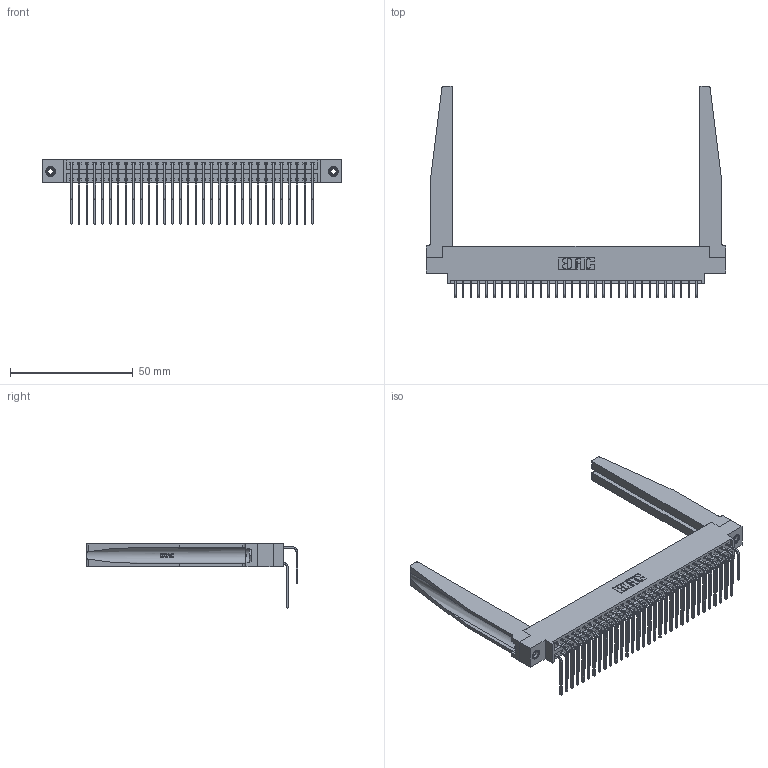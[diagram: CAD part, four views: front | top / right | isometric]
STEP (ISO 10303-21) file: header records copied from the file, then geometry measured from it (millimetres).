
FILE_DESCRIPTION (( 'STEP AP203' ), '1' );
FILE_NAME ('346-064-559-878.STEP', '2022-05-24T16:17:26', ( '' ), ( '' ), 'SwSTEP 2.0', 'SolidWorks 2020', '' );
FILE_SCHEMA (( 'CONFIG_CONTROL_DESIGN' ));
Length unit declared in the file: inch
Products named in the file (6): 346-220-078_345-220-078; 346-064-559-878; 346 Part_0.170 Offset - 0.156 Dia-TH; 345-250-001_345-250-001-102; 345-292-001_558 559 Tail - 1; 345-292-001_559 Tail - 2
Assembly tree (69 placements, depth 2):
  346-064-559-878
    346 Part_0.170 Offset - 0.156 Dia-TH
    345-292-001_558 559 Tail - 1  x32
    345-292-001_559 Tail - 2  x32
    346-220-078_345-220-078  x2
    345-250-001_345-250-001-102  x2
Bounding box: 122.17 x 86.17 x 26.16 mm (x, y, z)
Volume: 18941.2 mm3; surface area: 24904.9 mm2
Topology: 69 solids, 69 shells, 3830 faces, 11289 edges, 7430 vertices
Faces by surface type: plane 2604, cylinder 1174, bspline 36, cone 12, torus 4
Entity records: 29310 total; most frequent: CARTESIAN_POINT 5840, ORIENTED_EDGE 4610, DIRECTION 4155, EDGE_CURVE 2305, VECTOR 1911, LINE 1911, VERTEX_POINT 1528, AXIS2_PLACEMENT_3D 1122
